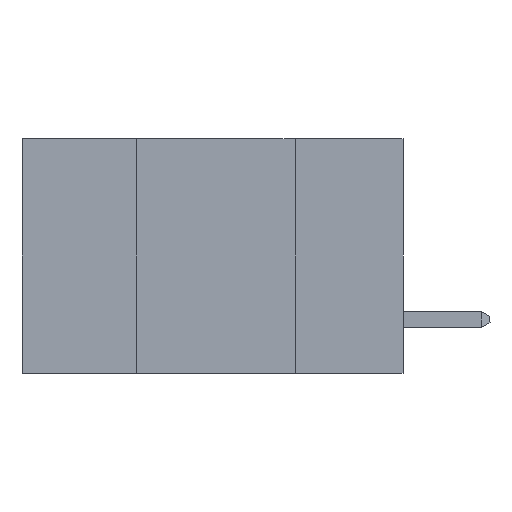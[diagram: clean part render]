
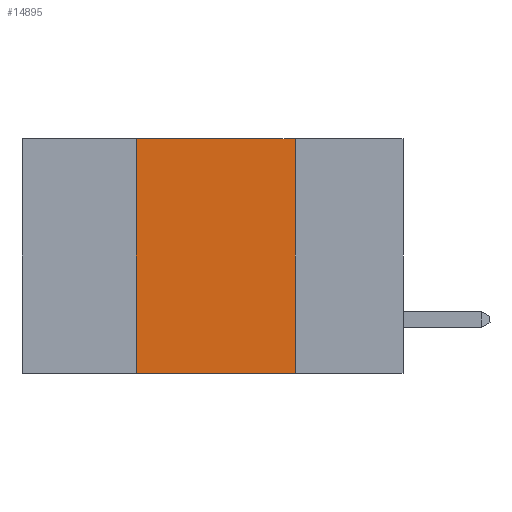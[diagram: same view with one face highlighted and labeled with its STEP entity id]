
A CAD part, left-side view. The second image highlights one B-rep face of the part: STEP entity #14895.
In plain terms, the highlighted planar face has unit normal (-1, 0, 0).
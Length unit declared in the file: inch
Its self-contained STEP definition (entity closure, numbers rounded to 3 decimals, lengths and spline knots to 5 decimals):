
#696 = EDGE_CURVE ( 'NONE', #11277, #17379, #19597, .T. ) ;
#852 = VERTEX_POINT ( 'NONE', #7113 ) ;
#1593 = ORIENTED_EDGE ( 'NONE', *, *, #3057, .F. ) ;
#1935 = LINE ( 'NONE', #7222, #13988 ) ;
#2105 = ORIENTED_EDGE ( 'NONE', *, *, #10660, .F. ) ;
#2862 = EDGE_CURVE ( 'NONE', #11277, #852, #9672, .T. ) ;
#3057 = EDGE_CURVE ( 'NONE', #852, #12712, #1935, .T. ) ;
#4010 = DIRECTION ( 'NONE',  ( 1., 0., 0. ) ) ;
#4893 = ORIENTED_EDGE ( 'NONE', *, *, #696, .T. ) ;
#7094 = PLANE ( 'NONE',  #9877 ) ;
#7113 = CARTESIAN_POINT ( 'NONE',  ( 0., 0.42, 0. ) ) ;
#7222 = CARTESIAN_POINT ( 'NONE',  ( 0., 0.6, 0. ) ) ;
#7430 = VECTOR ( 'NONE', #14748, 39.37008 ) ;
#7641 = DIRECTION ( 'NONE',  ( 0., -1., 0. ) ) ;
#9672 = LINE ( 'NONE', #10682, #13766 ) ;
#9877 = AXIS2_PLACEMENT_3D ( 'NONE', #11829, #4010, #14863 ) ;
#10206 = CARTESIAN_POINT ( 'NONE',  ( 0., 0.17, 0. ) ) ;
#10660 = EDGE_CURVE ( 'NONE', #12712, #17379, #11097, .T. ) ;
#10682 = CARTESIAN_POINT ( 'NONE',  ( 0., 0.42, 0. ) ) ;
#11097 = LINE ( 'NONE', #10206, #7430 ) ;
#11192 = VECTOR ( 'NONE', #18577, 39.37008 ) ;
#11277 = VERTEX_POINT ( 'NONE', #16029 ) ;
#11829 = CARTESIAN_POINT ( 'NONE',  ( 0., 0.6, 0. ) ) ;
#12159 = FACE_OUTER_BOUND ( 'NONE', #12324, .T. ) ;
#12324 = EDGE_LOOP ( 'NONE', ( #2105, #1593, #17655, #4893 ) ) ;
#12712 = VERTEX_POINT ( 'NONE', #16749 ) ;
#12721 = CARTESIAN_POINT ( 'NONE',  ( 0., 0.17, -0.37 ) ) ;
#13766 = VECTOR ( 'NONE', #17591, 39.37008 ) ;
#13988 = VECTOR ( 'NONE', #7641, 39.37008 ) ;
#14748 = DIRECTION ( 'NONE',  ( 0., 0., -1. ) ) ;
#14863 = DIRECTION ( 'NONE',  ( 0., 0., -1. ) ) ;
#14895 = ADVANCED_FACE ( 'NONE', ( #12159 ), #7094, .F. ) ;
#16029 = CARTESIAN_POINT ( 'NONE',  ( 0., 0.42, -0.37 ) ) ;
#16462 = CARTESIAN_POINT ( 'NONE',  ( 0., 0.6, -0.37 ) ) ;
#16749 = CARTESIAN_POINT ( 'NONE',  ( 0., 0.17, 0. ) ) ;
#17379 = VERTEX_POINT ( 'NONE', #12721 ) ;
#17591 = DIRECTION ( 'NONE',  ( 0., 0., 1. ) ) ;
#17655 = ORIENTED_EDGE ( 'NONE', *, *, #2862, .F. ) ;
#18577 = DIRECTION ( 'NONE',  ( 0., -1., 0. ) ) ;
#19597 = LINE ( 'NONE', #16462, #11192 ) ;
